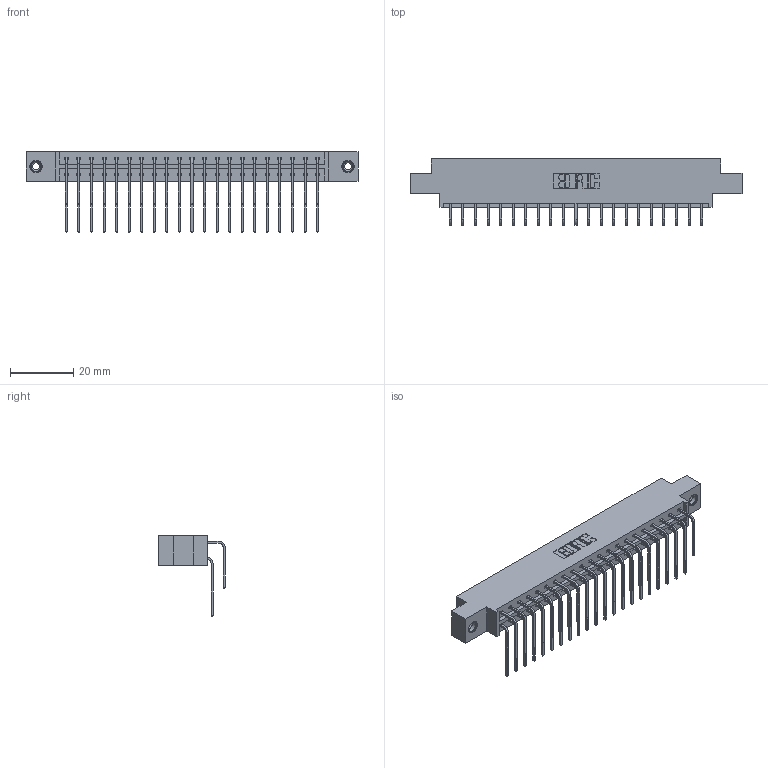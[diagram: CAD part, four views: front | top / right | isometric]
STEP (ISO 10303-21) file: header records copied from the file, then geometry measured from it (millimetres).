
FILE_DESCRIPTION (( 'STEP AP203' ), '1' );
FILE_NAME ('833-042-559-808.STEP', '2020-06-03T22:55:25', ( '' ), ( '' ), 'SwSTEP 2.0', 'SolidWorks 2020', '' );
FILE_SCHEMA (( 'CONFIG_CONTROL_DESIGN' ));
Length unit declared in the file: inch
Products named in the file (5): 345-250-001_345-250-003-102; 345-292-001_558 559 Tail - 1; 833-042-559-808; 833 Part_Offset - .156 Dia - TI; 345-292-001_559 Tail - 2
Assembly tree (45 placements, depth 2):
  833-042-559-808
    833 Part_Offset - .156 Dia - TI
    345-292-001_558 559 Tail - 1  x21
    345-292-001_559 Tail - 2  x21
    345-250-001_345-250-003-102  x2
Bounding box: 104.75 x 20.9 x 25.53 mm (x, y, z)
Volume: 10505.9 mm3; surface area: 13644.4 mm2
Topology: 45 solids, 45 shells, 2446 faces, 7221 edges, 4750 vertices
Faces by surface type: plane 1702, cylinder 728, cone 12, torus 4
Entity records: 19328 total; most frequent: CARTESIAN_POINT 3264, ORIENTED_EDGE 3142, DIRECTION 2837, EDGE_CURVE 1571, LINE 1383, VECTOR 1383, VERTEX_POINT 1040, AXIS2_PLACEMENT_3D 727
